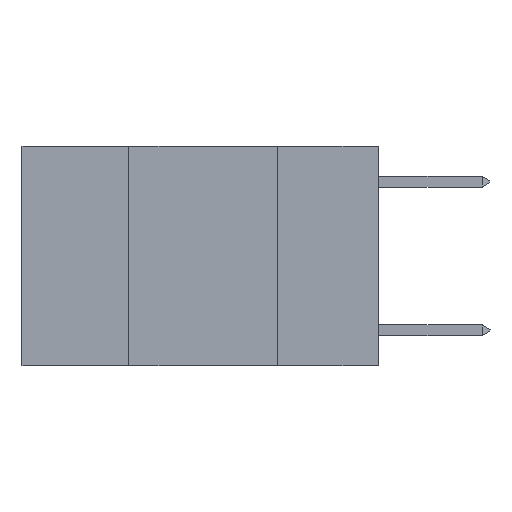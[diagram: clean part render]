
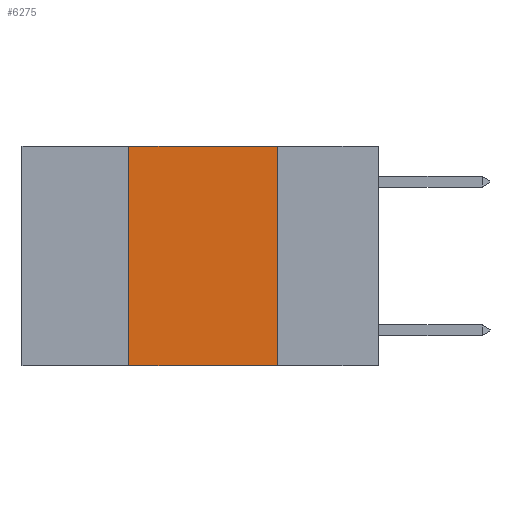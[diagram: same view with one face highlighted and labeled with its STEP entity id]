
A CAD part, left-side view. The second image highlights one B-rep face of the part: STEP entity #6275.
In plain terms, the highlighted planar face has unit normal (-1, 0, 0).
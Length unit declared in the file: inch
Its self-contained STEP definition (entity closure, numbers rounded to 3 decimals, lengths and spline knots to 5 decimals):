
#6 = VERTEX_POINT ( 'NONE', #7142 ) ;
#193 = CARTESIAN_POINT ( 'NONE',  ( 0., 0.17, -0.37 ) ) ;
#258 = VERTEX_POINT ( 'NONE', #2009 ) ;
#583 = CARTESIAN_POINT ( 'NONE',  ( 0., 0.6, 0. ) ) ;
#601 = CARTESIAN_POINT ( 'NONE',  ( 0., 0.6, -0.37 ) ) ;
#1300 = LINE ( 'NONE', #4740, #3475 ) ;
#2009 = CARTESIAN_POINT ( 'NONE',  ( 0., 0.17, 0. ) ) ;
#2203 = LINE ( 'NONE', #10052, #11495 ) ;
#2758 = CARTESIAN_POINT ( 'NONE',  ( 0., 0.6, 0. ) ) ;
#3432 = DIRECTION ( 'NONE',  ( 0., -1., 0. ) ) ;
#3475 = VECTOR ( 'NONE', #6573, 39.37008 ) ;
#3640 = VECTOR ( 'NONE', #3432, 39.37008 ) ;
#3666 = DIRECTION ( 'NONE',  ( 0., 0., -1. ) ) ;
#3867 = EDGE_CURVE ( 'NONE', #8346, #7233, #5364, .T. ) ;
#4290 = FACE_OUTER_BOUND ( 'NONE', #9714, .T. ) ;
#4447 = EDGE_CURVE ( 'NONE', #6, #258, #6344, .T. ) ;
#4740 = CARTESIAN_POINT ( 'NONE',  ( 0., 0.17, 0. ) ) ;
#5144 = ORIENTED_EDGE ( 'NONE', *, *, #3867, .T. ) ;
#5364 = LINE ( 'NONE', #601, #5650 ) ;
#5650 = VECTOR ( 'NONE', #7992, 39.37008 ) ;
#6275 = ADVANCED_FACE ( 'NONE', ( #4290 ), #8177, .F. ) ;
#6344 = LINE ( 'NONE', #583, #3640 ) ;
#6490 = DIRECTION ( 'NONE',  ( 0., 0., 1. ) ) ;
#6573 = DIRECTION ( 'NONE',  ( 0., 0., -1. ) ) ;
#7142 = CARTESIAN_POINT ( 'NONE',  ( 0., 0.42, 0. ) ) ;
#7233 = VERTEX_POINT ( 'NONE', #193 ) ;
#7992 = DIRECTION ( 'NONE',  ( 0., -1., 0. ) ) ;
#8073 = AXIS2_PLACEMENT_3D ( 'NONE', #2758, #9094, #3666 ) ;
#8177 = PLANE ( 'NONE',  #8073 ) ;
#8346 = VERTEX_POINT ( 'NONE', #9524 ) ;
#8475 = ORIENTED_EDGE ( 'NONE', *, *, #10774, .F. ) ;
#8829 = ORIENTED_EDGE ( 'NONE', *, *, #4447, .F. ) ;
#9094 = DIRECTION ( 'NONE',  ( 1., 0., 0. ) ) ;
#9524 = CARTESIAN_POINT ( 'NONE',  ( 0., 0.42, -0.37 ) ) ;
#9714 = EDGE_LOOP ( 'NONE', ( #10973, #8829, #8475, #5144 ) ) ;
#10052 = CARTESIAN_POINT ( 'NONE',  ( 0., 0.42, 0. ) ) ;
#10774 = EDGE_CURVE ( 'NONE', #8346, #6, #2203, .T. ) ;
#10973 = ORIENTED_EDGE ( 'NONE', *, *, #11377, .F. ) ;
#11377 = EDGE_CURVE ( 'NONE', #258, #7233, #1300, .T. ) ;
#11495 = VECTOR ( 'NONE', #6490, 39.37008 ) ;
